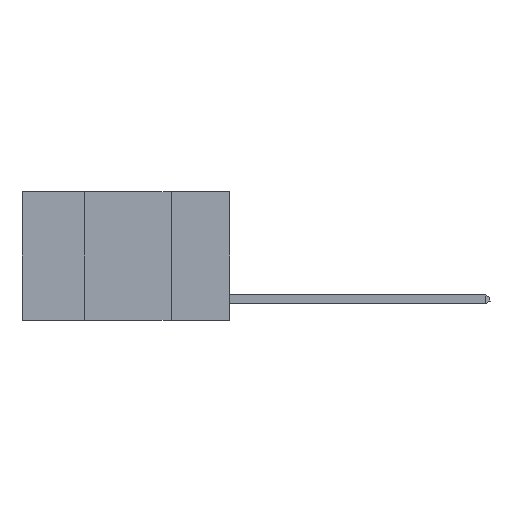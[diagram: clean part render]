
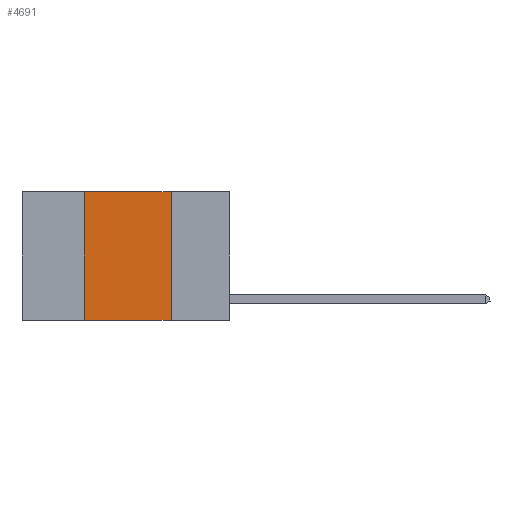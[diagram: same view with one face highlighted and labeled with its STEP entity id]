
A CAD part, left-side view. The second image highlights one B-rep face of the part: STEP entity #4691.
In plain terms, the highlighted planar face has unit normal (-1, 0, 0).
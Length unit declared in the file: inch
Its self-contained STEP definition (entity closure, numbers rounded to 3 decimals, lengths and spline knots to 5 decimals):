
#365 = DIRECTION ( 'NONE',  ( 0., 0., 1. ) ) ;
#688 = VERTEX_POINT ( 'NONE', #799 ) ;
#799 = CARTESIAN_POINT ( 'NONE',  ( 0., 0.17, -0.37 ) ) ;
#1136 = LINE ( 'NONE', #11298, #12816 ) ;
#1147 = DIRECTION ( 'NONE',  ( 0., 0., -1. ) ) ;
#1308 = ORIENTED_EDGE ( 'NONE', *, *, #7802, .T. ) ;
#1700 = EDGE_CURVE ( 'NONE', #7877, #11047, #1136, .T. ) ;
#1765 = AXIS2_PLACEMENT_3D ( 'NONE', #11519, #4771, #12615 ) ;
#2667 = ORIENTED_EDGE ( 'NONE', *, *, #11816, .F. ) ;
#2673 = LINE ( 'NONE', #8406, #12377 ) ;
#2762 = CARTESIAN_POINT ( 'NONE',  ( 0., 0.42, -0.37 ) ) ;
#2964 = LINE ( 'NONE', #4216, #11650 ) ;
#4216 = CARTESIAN_POINT ( 'NONE',  ( 0., 0.6, -0.37 ) ) ;
#4691 = ADVANCED_FACE ( 'NONE', ( #5019 ), #11471, .F. ) ;
#4771 = DIRECTION ( 'NONE',  ( 1., 0., 0. ) ) ;
#5019 = FACE_OUTER_BOUND ( 'NONE', #7118, .T. ) ;
#5663 = VECTOR ( 'NONE', #1147, 39.37008 ) ;
#6032 = LINE ( 'NONE', #9167, #5663 ) ;
#7118 = EDGE_LOOP ( 'NONE', ( #12965, #7829, #2667, #1308 ) ) ;
#7802 = EDGE_CURVE ( 'NONE', #12798, #688, #2964, .T. ) ;
#7829 = ORIENTED_EDGE ( 'NONE', *, *, #1700, .F. ) ;
#7877 = VERTEX_POINT ( 'NONE', #10036 ) ;
#8406 = CARTESIAN_POINT ( 'NONE',  ( 0., 0.42, 0. ) ) ;
#9167 = CARTESIAN_POINT ( 'NONE',  ( 0., 0.17, 0. ) ) ;
#10036 = CARTESIAN_POINT ( 'NONE',  ( 0., 0.42, 0. ) ) ;
#10576 = DIRECTION ( 'NONE',  ( 0., -1., 0. ) ) ;
#11007 = DIRECTION ( 'NONE',  ( 0., -1., 0. ) ) ;
#11047 = VERTEX_POINT ( 'NONE', #13738 ) ;
#11298 = CARTESIAN_POINT ( 'NONE',  ( 0., 0.6, 0. ) ) ;
#11471 = PLANE ( 'NONE',  #1765 ) ;
#11519 = CARTESIAN_POINT ( 'NONE',  ( 0., 0.6, 0. ) ) ;
#11650 = VECTOR ( 'NONE', #11007, 39.37008 ) ;
#11816 = EDGE_CURVE ( 'NONE', #12798, #7877, #2673, .T. ) ;
#12377 = VECTOR ( 'NONE', #365, 39.37008 ) ;
#12615 = DIRECTION ( 'NONE',  ( 0., 0., -1. ) ) ;
#12798 = VERTEX_POINT ( 'NONE', #2762 ) ;
#12816 = VECTOR ( 'NONE', #10576, 39.37008 ) ;
#12965 = ORIENTED_EDGE ( 'NONE', *, *, #14500, .F. ) ;
#13738 = CARTESIAN_POINT ( 'NONE',  ( 0., 0.17, 0. ) ) ;
#14500 = EDGE_CURVE ( 'NONE', #11047, #688, #6032, .T. ) ;
